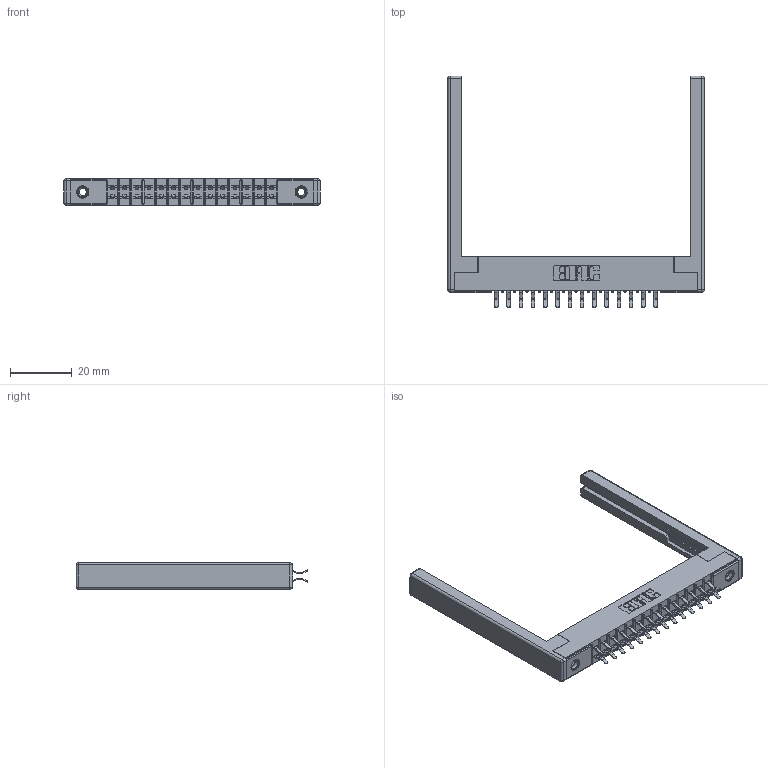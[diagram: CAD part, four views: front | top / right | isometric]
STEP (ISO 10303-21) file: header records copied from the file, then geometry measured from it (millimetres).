
FILE_DESCRIPTION (( 'STEP AP203' ), '1' );
FILE_NAME ('355-028-556-268.STEP', '2019-09-11T06:40:16', ( '' ), ( '' ), 'SwSTEP 2.0', 'SolidWorks 2016', '' );
FILE_SCHEMA (( 'CONFIG_CONTROL_DESIGN' ));
Length unit declared in the file: inch
Products named in the file (5): 345-250-001_345-250-001-102; 355-028-556-268; 305-290-001_556; 305 Part_.156 Dia; 307-220-068
Assembly tree (33 placements, depth 2):
  355-028-556-268
    305 Part_.156 Dia
    305-290-001_556  x28
    345-250-001_345-250-001-102  x2
    307-220-068  x2
Bounding box: 82.91 x 74.93 x 8.71 mm (x, y, z)
Volume: 9776.9 mm3; surface area: 13408.3 mm2
Topology: 33 solids, 33 shells, 1838 faces, 5228 edges, 3388 vertices
Faces by surface type: plane 1024, cylinder 734, sphere 64, cone 12, torus 4
Entity records: 21548 total; most frequent: CARTESIAN_POINT 3541, ORIENTED_EDGE 3502, DIRECTION 3471, EDGE_CURVE 1751, LINE 1371, VECTOR 1371, VERTEX_POINT 1120, AXIS2_PLACEMENT_3D 1050
